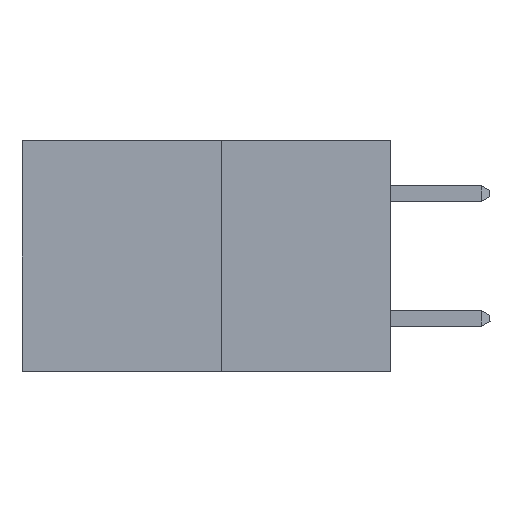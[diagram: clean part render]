
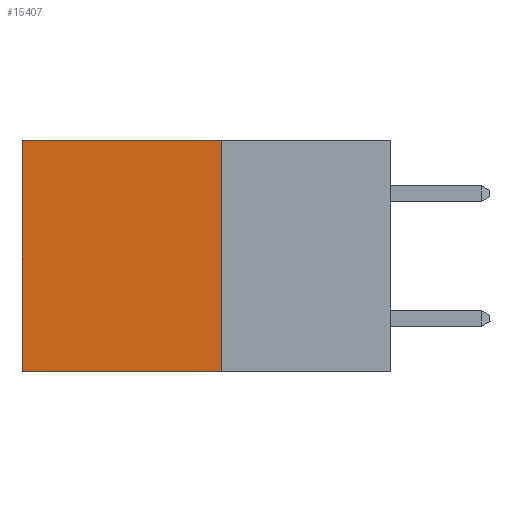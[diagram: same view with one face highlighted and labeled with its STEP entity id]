
A CAD part, left-side view. The second image highlights one B-rep face of the part: STEP entity #15407.
In plain terms, the highlighted planar face has unit normal (-1, 0, 0).
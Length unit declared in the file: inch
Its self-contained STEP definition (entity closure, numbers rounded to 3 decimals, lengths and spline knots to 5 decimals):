
#3 = CARTESIAN_POINT ( 'NONE',  ( 0.277, 0.59, -0.37 ) ) ;
#930 = CARTESIAN_POINT ( 'NONE',  ( 0.277, 0.27, -0.37 ) ) ;
#1143 = DIRECTION ( 'NONE',  ( 0., 1., 0. ) ) ;
#1510 = DIRECTION ( 'NONE',  ( 0., 0., -1. ) ) ;
#2257 = EDGE_CURVE ( 'NONE', #10642, #13468, #12895, .T. ) ;
#2591 = VERTEX_POINT ( 'NONE', #22737 ) ;
#3194 = AXIS2_PLACEMENT_3D ( 'NONE', #6775, #22203, #10675 ) ;
#4805 = EDGE_CURVE ( 'NONE', #2591, #13468, #21857, .T. ) ;
#5410 = EDGE_CURVE ( 'NONE', #20982, #10642, #8542, .T. ) ;
#6775 = CARTESIAN_POINT ( 'NONE',  ( 0.277, 0.27, -0.37 ) ) ;
#8108 = VECTOR ( 'NONE', #17004, 39.37008 ) ;
#8542 = LINE ( 'NONE', #10361, #13074 ) ;
#10124 = FACE_OUTER_BOUND ( 'NONE', #22260, .T. ) ;
#10361 = CARTESIAN_POINT ( 'NONE',  ( 0.277, 0.27, 0. ) ) ;
#10642 = VERTEX_POINT ( 'NONE', #16295 ) ;
#10675 = DIRECTION ( 'NONE',  ( 0., 0., -1. ) ) ;
#11822 = VECTOR ( 'NONE', #1510, 39.37008 ) ;
#12040 = EDGE_CURVE ( 'NONE', #20982, #2591, #16297, .T. ) ;
#12522 = ORIENTED_EDGE ( 'NONE', *, *, #2257, .T. ) ;
#12895 = LINE ( 'NONE', #24812, #8108 ) ;
#13074 = VECTOR ( 'NONE', #16148, 39.37008 ) ;
#13110 = CARTESIAN_POINT ( 'NONE',  ( 0.277, 0.27, -0.37 ) ) ;
#13468 = VERTEX_POINT ( 'NONE', #3 ) ;
#14664 = ORIENTED_EDGE ( 'NONE', *, *, #12040, .F. ) ;
#15407 = ADVANCED_FACE ( 'NONE', ( #10124 ), #20283, .F. ) ;
#16148 = DIRECTION ( 'NONE',  ( 0., 1., 0. ) ) ;
#16243 = ORIENTED_EDGE ( 'NONE', *, *, #5410, .T. ) ;
#16295 = CARTESIAN_POINT ( 'NONE',  ( 0.277, 0.59, 0. ) ) ;
#16297 = LINE ( 'NONE', #13110, #11822 ) ;
#16706 = VECTOR ( 'NONE', #1143, 39.37008 ) ;
#17004 = DIRECTION ( 'NONE',  ( 0., 0., -1. ) ) ;
#17306 = CARTESIAN_POINT ( 'NONE',  ( 0.277, 0.27, 0. ) ) ;
#18944 = ORIENTED_EDGE ( 'NONE', *, *, #4805, .F. ) ;
#20283 = PLANE ( 'NONE',  #3194 ) ;
#20982 = VERTEX_POINT ( 'NONE', #17306 ) ;
#21857 = LINE ( 'NONE', #930, #16706 ) ;
#22203 = DIRECTION ( 'NONE',  ( 1., 0., 0. ) ) ;
#22260 = EDGE_LOOP ( 'NONE', ( #12522, #18944, #14664, #16243 ) ) ;
#22737 = CARTESIAN_POINT ( 'NONE',  ( 0.277, 0.27, -0.37 ) ) ;
#24812 = CARTESIAN_POINT ( 'NONE',  ( 0.277, 0.59, -0.37 ) ) ;
